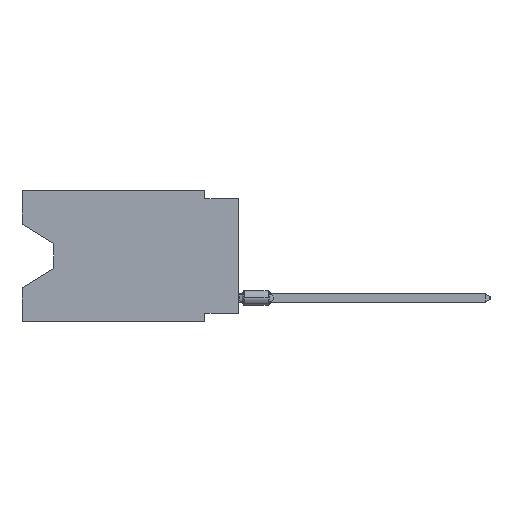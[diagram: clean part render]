
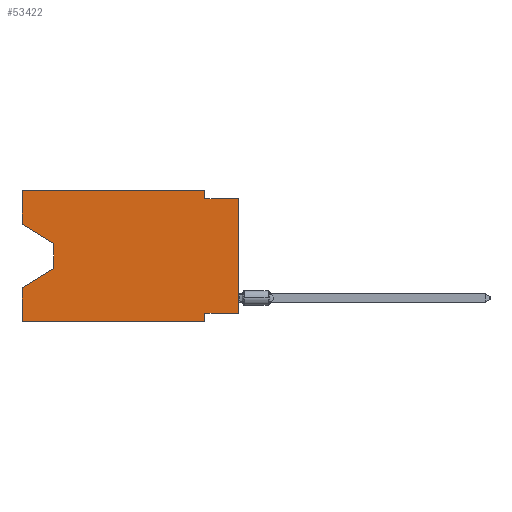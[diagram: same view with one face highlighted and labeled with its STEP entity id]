
A CAD part, left-side view. The second image highlights one B-rep face of the part: STEP entity #53422.
In plain terms, the highlighted planar face has unit normal (-1, 0, 0).
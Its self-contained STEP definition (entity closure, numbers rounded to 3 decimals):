
#504 = EDGE_CURVE ( 'NONE', #17596, #62265, #11219, .T. ) ;
#1084 = CARTESIAN_POINT ( 'NONE',  ( 0., 13.97, -4.013 ) ) ;
#1906 = EDGE_CURVE ( 'NONE', #13272, #45729, #49112, .T. ) ;
#2474 = CARTESIAN_POINT ( 'NONE',  ( 0., 2.54, 0. ) ) ;
#3244 = DIRECTION ( 'NONE',  ( 0., 1., 0. ) ) ;
#4204 = VERTEX_POINT ( 'NONE', #22548 ) ;
#4827 = ORIENTED_EDGE ( 'NONE', *, *, #24185, .T. ) ;
#5156 = CARTESIAN_POINT ( 'NONE',  ( 0., 16.383, 0. ) ) ;
#5989 = CARTESIAN_POINT ( 'NONE',  ( 0., 13.97, -5.893 ) ) ;
#6771 = DIRECTION ( 'NONE',  ( 0., 0., -1. ) ) ;
#7987 = VECTOR ( 'NONE', #44975, 1000. ) ;
#8479 = CARTESIAN_POINT ( 'NONE',  ( 0., 13.97, -5.893 ) ) ;
#9553 = PLANE ( 'NONE',  #47392 ) ;
#9996 = LINE ( 'NONE', #14687, #59441 ) ;
#10023 = EDGE_CURVE ( 'NONE', #52662, #4204, #44503, .T. ) ;
#10536 = VECTOR ( 'NONE', #30984, 1000. ) ;
#10732 = VECTOR ( 'NONE', #55707, 1000. ) ;
#11219 = LINE ( 'NONE', #11546, #10536 ) ;
#11299 = VERTEX_POINT ( 'NONE', #14347 ) ;
#11385 = LINE ( 'NONE', #41532, #17335 ) ;
#11546 = CARTESIAN_POINT ( 'NONE',  ( 0., 16.383, 0. ) ) ;
#12105 = LINE ( 'NONE', #1084, #19076 ) ;
#12858 = EDGE_CURVE ( 'NONE', #4204, #42185, #12105, .T. ) ;
#12934 = ORIENTED_EDGE ( 'NONE', *, *, #504, .F. ) ;
#13272 = VERTEX_POINT ( 'NONE', #23059 ) ;
#13876 = CARTESIAN_POINT ( 'NONE',  ( 0., 0., -0.635 ) ) ;
#14006 = DIRECTION ( 'NONE',  ( 0., -0.855, -0.519 ) ) ;
#14229 = FACE_OUTER_BOUND ( 'NONE', #34483, .T. ) ;
#14347 = CARTESIAN_POINT ( 'NONE',  ( 0., 16.383, -7.36 ) ) ;
#14687 = CARTESIAN_POINT ( 'NONE',  ( 0., 0., -0.635 ) ) ;
#15057 = EDGE_CURVE ( 'NONE', #52662, #17596, #50688, .T. ) ;
#15880 = VERTEX_POINT ( 'NONE', #33640 ) ;
#16364 = EDGE_CURVE ( 'NONE', #45307, #11299, #39910, .T. ) ;
#16463 = ORIENTED_EDGE ( 'NONE', *, *, #16364, .F. ) ;
#17335 = VECTOR ( 'NONE', #51575, 1000. ) ;
#17596 = VERTEX_POINT ( 'NONE', #22610 ) ;
#18369 = CARTESIAN_POINT ( 'NONE',  ( 0., 16.383, -2.546 ) ) ;
#19076 = VECTOR ( 'NONE', #6771, 1000. ) ;
#20177 = DIRECTION ( 'NONE',  ( 0., 0.855, -0.519 ) ) ;
#22548 = CARTESIAN_POINT ( 'NONE',  ( 0., 13.97, -4.013 ) ) ;
#22610 = CARTESIAN_POINT ( 'NONE',  ( 0., 16.383, 0. ) ) ;
#22986 = CARTESIAN_POINT ( 'NONE',  ( 0., 0., -9.271 ) ) ;
#23059 = CARTESIAN_POINT ( 'NONE',  ( 0., 0., -9.271 ) ) ;
#23500 = DIRECTION ( 'NONE',  ( 0., 0., 1. ) ) ;
#24185 = EDGE_CURVE ( 'NONE', #42185, #11299, #33922, .T. ) ;
#24190 = CARTESIAN_POINT ( 'NONE',  ( 0., 16.383, -2.546 ) ) ;
#24274 = DIRECTION ( 'NONE',  ( 0., 0., -1. ) ) ;
#24694 = ORIENTED_EDGE ( 'NONE', *, *, #26842, .T. ) ;
#25574 = DIRECTION ( 'NONE',  ( 0., 0., -1. ) ) ;
#26842 = EDGE_CURVE ( 'NONE', #13272, #49305, #54340, .T. ) ;
#27413 = VECTOR ( 'NONE', #14006, 1000. ) ;
#27822 = ORIENTED_EDGE ( 'NONE', *, *, #10023, .T. ) ;
#28846 = LINE ( 'NONE', #49938, #35149 ) ;
#30633 = CARTESIAN_POINT ( 'NONE',  ( 0., 16.383, 0. ) ) ;
#30725 = ORIENTED_EDGE ( 'NONE', *, *, #12858, .T. ) ;
#30984 = DIRECTION ( 'NONE',  ( 0., -1., 0. ) ) ;
#32570 = ORIENTED_EDGE ( 'NONE', *, *, #15057, .F. ) ;
#33562 = CARTESIAN_POINT ( 'NONE',  ( 0., 16.383, 0. ) ) ;
#33640 = CARTESIAN_POINT ( 'NONE',  ( 0., 2.54, -0.635 ) ) ;
#33922 = LINE ( 'NONE', #8479, #42244 ) ;
#33991 = ORIENTED_EDGE ( 'NONE', *, *, #44703, .F. ) ;
#34483 = EDGE_LOOP ( 'NONE', ( #27822, #30725, #4827, #16463, #35317, #38821, #66035, #24694, #33991, #34541, #12934, #32570 ) ) ;
#34541 = ORIENTED_EDGE ( 'NONE', *, *, #49283, .F. ) ;
#34659 = DIRECTION ( 'NONE',  ( 1., 0., 0. ) ) ;
#35149 = VECTOR ( 'NONE', #65008, 1000. ) ;
#35317 = ORIENTED_EDGE ( 'NONE', *, *, #61974, .T. ) ;
#36496 = VECTOR ( 'NONE', #23500, 1000. ) ;
#38821 = ORIENTED_EDGE ( 'NONE', *, *, #54313, .F. ) ;
#38938 = CARTESIAN_POINT ( 'NONE',  ( 0., 0., 0. ) ) ;
#39656 = LINE ( 'NONE', #39986, #61945 ) ;
#39910 = LINE ( 'NONE', #33562, #36496 ) ;
#39986 = CARTESIAN_POINT ( 'NONE',  ( 0., 2.54, 0. ) ) ;
#41532 = CARTESIAN_POINT ( 'NONE',  ( 0., 2.54, -9.906 ) ) ;
#41725 = CARTESIAN_POINT ( 'NONE',  ( 0., 16.383, -9.906 ) ) ;
#42185 = VERTEX_POINT ( 'NONE', #5989 ) ;
#42244 = VECTOR ( 'NONE', #20177, 1000. ) ;
#43810 = VECTOR ( 'NONE', #3244, 1000. ) ;
#44503 = LINE ( 'NONE', #18369, #27413 ) ;
#44703 = EDGE_CURVE ( 'NONE', #15880, #49305, #9996, .T. ) ;
#44975 = DIRECTION ( 'NONE',  ( 0., 0., 1. ) ) ;
#45307 = VERTEX_POINT ( 'NONE', #41725 ) ;
#45729 = VERTEX_POINT ( 'NONE', #55373 ) ;
#47392 = AXIS2_PLACEMENT_3D ( 'NONE', #30633, #34659, #24274 ) ;
#49112 = LINE ( 'NONE', #22986, #43810 ) ;
#49283 = EDGE_CURVE ( 'NONE', #62265, #15880, #39656, .T. ) ;
#49305 = VERTEX_POINT ( 'NONE', #13876 ) ;
#49919 = VERTEX_POINT ( 'NONE', #58849 ) ;
#49938 = CARTESIAN_POINT ( 'NONE',  ( 0., 16.383, -9.906 ) ) ;
#50688 = LINE ( 'NONE', #5156, #10732 ) ;
#51575 = DIRECTION ( 'NONE',  ( 0., 0., -1. ) ) ;
#52662 = VERTEX_POINT ( 'NONE', #24190 ) ;
#53422 = ADVANCED_FACE ( 'NONE', ( #14229 ), #9553, .F. ) ;
#54313 = EDGE_CURVE ( 'NONE', #45729, #49919, #11385, .T. ) ;
#54340 = LINE ( 'NONE', #38938, #7987 ) ;
#55373 = CARTESIAN_POINT ( 'NONE',  ( 0., 2.54, -9.271 ) ) ;
#55707 = DIRECTION ( 'NONE',  ( 0., 0., 1. ) ) ;
#55872 = DIRECTION ( 'NONE',  ( 0., -1., 0. ) ) ;
#58849 = CARTESIAN_POINT ( 'NONE',  ( 0., 2.54, -9.906 ) ) ;
#59441 = VECTOR ( 'NONE', #55872, 1000. ) ;
#61945 = VECTOR ( 'NONE', #25574, 1000. ) ;
#61974 = EDGE_CURVE ( 'NONE', #45307, #49919, #28846, .T. ) ;
#62265 = VERTEX_POINT ( 'NONE', #2474 ) ;
#65008 = DIRECTION ( 'NONE',  ( 0., -1., 0. ) ) ;
#66035 = ORIENTED_EDGE ( 'NONE', *, *, #1906, .F. ) ;
